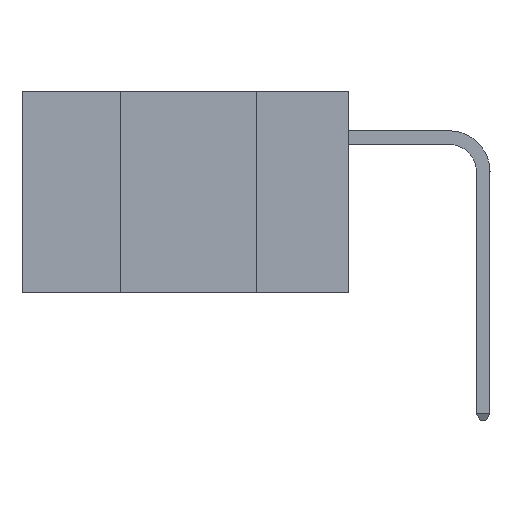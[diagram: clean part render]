
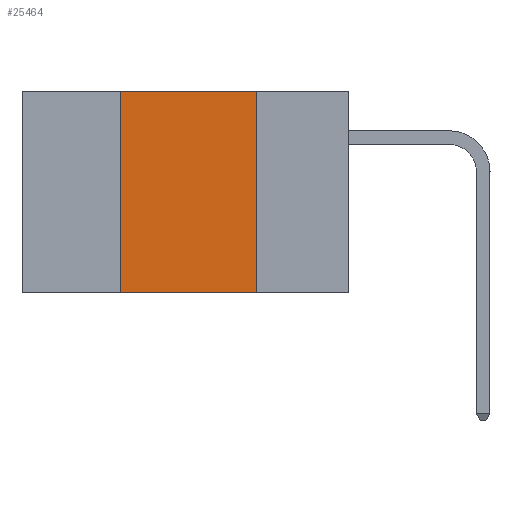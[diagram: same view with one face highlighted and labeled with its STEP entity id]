
A CAD part, left-side view. The second image highlights one B-rep face of the part: STEP entity #25464.
In plain terms, the highlighted planar face has unit normal (-1, 0, 0).
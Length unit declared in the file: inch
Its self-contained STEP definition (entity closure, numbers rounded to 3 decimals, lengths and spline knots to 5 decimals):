
#536 = CARTESIAN_POINT ( 'NONE',  ( 0., 0.6, -0.37 ) ) ;
#2046 = PLANE ( 'NONE',  #7721 ) ;
#2386 = LINE ( 'NONE', #35206, #24520 ) ;
#2588 = VECTOR ( 'NONE', #24581, 39.37008 ) ;
#2689 = EDGE_CURVE ( 'NONE', #13429, #9383, #25620, .T. ) ;
#3178 = ORIENTED_EDGE ( 'NONE', *, *, #31528, .T. ) ;
#3454 = DIRECTION ( 'NONE',  ( 0., -1., 0. ) ) ;
#3573 = DIRECTION ( 'NONE',  ( 0., 0., -1. ) ) ;
#4942 = ORIENTED_EDGE ( 'NONE', *, *, #2689, .F. ) ;
#4953 = DIRECTION ( 'NONE',  ( 1., 0., 0. ) ) ;
#5161 = LINE ( 'NONE', #11657, #27296 ) ;
#7023 = CARTESIAN_POINT ( 'NONE',  ( 0., 0.42, -0.37 ) ) ;
#7369 = VERTEX_POINT ( 'NONE', #29812 ) ;
#7721 = AXIS2_PLACEMENT_3D ( 'NONE', #27930, #4953, #25119 ) ;
#9156 = CARTESIAN_POINT ( 'NONE',  ( 0., 0.17, 0. ) ) ;
#9383 = VERTEX_POINT ( 'NONE', #9156 ) ;
#11657 = CARTESIAN_POINT ( 'NONE',  ( 0., 0.42, 0. ) ) ;
#13429 = VERTEX_POINT ( 'NONE', #14847 ) ;
#14471 = DIRECTION ( 'NONE',  ( 0., 0., 1. ) ) ;
#14847 = CARTESIAN_POINT ( 'NONE',  ( 0., 0.42, 0. ) ) ;
#16429 = VECTOR ( 'NONE', #3454, 39.37008 ) ;
#18094 = EDGE_CURVE ( 'NONE', #9383, #7369, #2386, .T. ) ;
#19226 = ORIENTED_EDGE ( 'NONE', *, *, #21941, .F. ) ;
#19577 = VERTEX_POINT ( 'NONE', #7023 ) ;
#21748 = CARTESIAN_POINT ( 'NONE',  ( 0., 0.6, 0. ) ) ;
#21941 = EDGE_CURVE ( 'NONE', #19577, #13429, #5161, .T. ) ;
#24048 = LINE ( 'NONE', #536, #16429 ) ;
#24520 = VECTOR ( 'NONE', #3573, 39.37008 ) ;
#24581 = DIRECTION ( 'NONE',  ( 0., -1., 0. ) ) ;
#25119 = DIRECTION ( 'NONE',  ( 0., 0., -1. ) ) ;
#25210 = ORIENTED_EDGE ( 'NONE', *, *, #18094, .F. ) ;
#25464 = ADVANCED_FACE ( 'NONE', ( #27957 ), #2046, .F. ) ;
#25620 = LINE ( 'NONE', #21748, #2588 ) ;
#27296 = VECTOR ( 'NONE', #14471, 39.37008 ) ;
#27930 = CARTESIAN_POINT ( 'NONE',  ( 0., 0.6, 0. ) ) ;
#27957 = FACE_OUTER_BOUND ( 'NONE', #36044, .T. ) ;
#29812 = CARTESIAN_POINT ( 'NONE',  ( 0., 0.17, -0.37 ) ) ;
#31528 = EDGE_CURVE ( 'NONE', #19577, #7369, #24048, .T. ) ;
#35206 = CARTESIAN_POINT ( 'NONE',  ( 0., 0.17, 0. ) ) ;
#36044 = EDGE_LOOP ( 'NONE', ( #25210, #4942, #19226, #3178 ) ) ;
